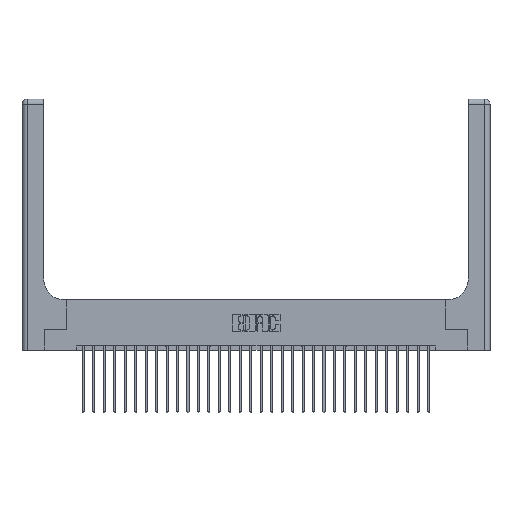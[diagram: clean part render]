
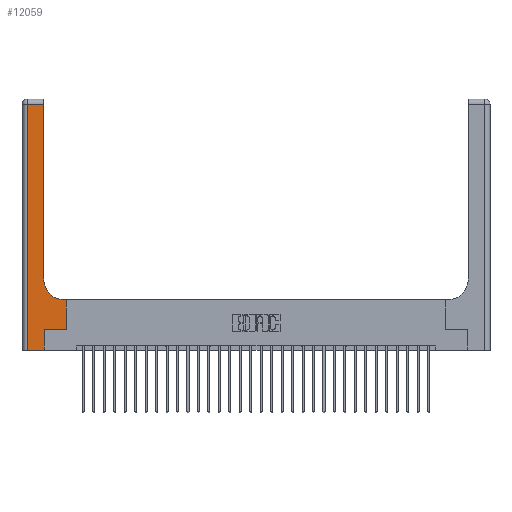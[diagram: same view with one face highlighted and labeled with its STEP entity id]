
A CAD part, top view. The second image highlights one B-rep face of the part: STEP entity #12059.
In plain terms, the highlighted planar face has unit normal (0, 0, 1).
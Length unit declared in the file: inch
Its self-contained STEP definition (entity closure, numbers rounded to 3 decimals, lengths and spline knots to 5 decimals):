
#55 = VECTOR ( 'NONE', #26331, 39.37008 ) ;
#72 = VECTOR ( 'NONE', #21310, 39.37008 ) ;
#436 = ORIENTED_EDGE ( 'NONE', *, *, #23866, .T. ) ;
#714 = DIRECTION ( 'NONE',  ( -1., 0., 0. ) ) ;
#1116 = VECTOR ( 'NONE', #714, 39.37008 ) ;
#1764 = CARTESIAN_POINT ( 'NONE',  ( 0.06, 3., 0.37 ) ) ;
#2154 = LINE ( 'NONE', #19172, #72 ) ;
#3018 = EDGE_CURVE ( 'NONE', #22150, #5124, #15526, .T. ) ;
#3043 = ORIENTED_EDGE ( 'NONE', *, *, #27311, .T. ) ;
#3549 = CARTESIAN_POINT ( 'NONE',  ( 0.26, 0.85, 0.37 ) ) ;
#3781 = CARTESIAN_POINT ( 'NONE',  ( 0.51, 0.85, 0.37 ) ) ;
#4613 = CARTESIAN_POINT ( 'NONE',  ( 0.265, 0., 0.37 ) ) ;
#4993 = DIRECTION ( 'NONE',  ( 0., 1., 0. ) ) ;
#5124 = VERTEX_POINT ( 'NONE', #4613 ) ;
#5157 = CARTESIAN_POINT ( 'NONE',  ( 0.06, 0., 0.37 ) ) ;
#5396 = LINE ( 'NONE', #1764, #17727 ) ;
#5740 = DIRECTION ( 'NONE',  ( 0., 1., 0. ) ) ;
#6293 = ORIENTED_EDGE ( 'NONE', *, *, #20589, .T. ) ;
#6613 = LINE ( 'NONE', #21767, #55 ) ;
#7165 = CARTESIAN_POINT ( 'NONE',  ( 0.26, 0.6, 0.37 ) ) ;
#7364 = CARTESIAN_POINT ( 'NONE',  ( 0.26, 2.94, 0.37 ) ) ;
#7714 = DIRECTION ( 'NONE',  ( 1., 0., 0. ) ) ;
#8319 = ORIENTED_EDGE ( 'NONE', *, *, #24906, .T. ) ;
#8656 = CARTESIAN_POINT ( 'NONE',  ( 0., 3., 0.37 ) ) ;
#9081 = DIRECTION ( 'NONE',  ( -1., 0., 0. ) ) ;
#9503 = ORIENTED_EDGE ( 'NONE', *, *, #3018, .T. ) ;
#11969 = CARTESIAN_POINT ( 'NONE',  ( 0.265, 0.25, 0.37 ) ) ;
#12059 = ADVANCED_FACE ( 'NONE', ( #12365 ), #17555, .F. ) ;
#12365 = FACE_OUTER_BOUND ( 'NONE', #21639, .T. ) ;
#12831 = VERTEX_POINT ( 'NONE', #17011 ) ;
#13484 = LINE ( 'NONE', #26593, #18598 ) ;
#14391 = VERTEX_POINT ( 'NONE', #7364 ) ;
#14544 = VERTEX_POINT ( 'NONE', #11969 ) ;
#14594 = CARTESIAN_POINT ( 'NONE',  ( 0., 0., 0.37 ) ) ;
#14721 = DIRECTION ( 'NONE',  ( 0., 0., -1. ) ) ;
#15526 = LINE ( 'NONE', #14594, #24172 ) ;
#15641 = LINE ( 'NONE', #23110, #21147 ) ;
#15706 = ORIENTED_EDGE ( 'NONE', *, *, #27822, .T. ) ;
#15832 = LINE ( 'NONE', #7165, #1116 ) ;
#15925 = EDGE_CURVE ( 'NONE', #14544, #12831, #6613, .T. ) ;
#17011 = CARTESIAN_POINT ( 'NONE',  ( 0.528, 0.25, 0.37 ) ) ;
#17208 = DIRECTION ( 'NONE',  ( 0., -1., 0. ) ) ;
#17555 = PLANE ( 'NONE',  #25112 ) ;
#17593 = CARTESIAN_POINT ( 'NONE',  ( 0.528, 0.6, 0.37 ) ) ;
#17727 = VECTOR ( 'NONE', #17208, 39.37008 ) ;
#17891 = CIRCLE ( 'NONE', #23063, 0.25 ) ;
#18023 = DIRECTION ( 'NONE',  ( 0., 0., -1. ) ) ;
#18598 = VECTOR ( 'NONE', #9081, 39.37008 ) ;
#19172 = CARTESIAN_POINT ( 'NONE',  ( 0.265, 0., 0.37 ) ) ;
#20398 = ORIENTED_EDGE ( 'NONE', *, *, #15925, .T. ) ;
#20431 = DIRECTION ( 'NONE',  ( -1., 0., 0. ) ) ;
#20589 = EDGE_CURVE ( 'NONE', #26113, #14391, #15641, .T. ) ;
#21147 = VECTOR ( 'NONE', #5740, 39.37008 ) ;
#21310 = DIRECTION ( 'NONE',  ( 0., 1., 0. ) ) ;
#21639 = EDGE_LOOP ( 'NONE', ( #6293, #436, #8319, #9503, #3043, #20398, #26735, #26748, #15706 ) ) ;
#21767 = CARTESIAN_POINT ( 'NONE',  ( 0.265, 0.25, 0.37 ) ) ;
#22150 = VERTEX_POINT ( 'NONE', #5157 ) ;
#22161 = CARTESIAN_POINT ( 'NONE',  ( 0.528, 0.25, 0.37 ) ) ;
#23063 = AXIS2_PLACEMENT_3D ( 'NONE', #3781, #14721, #26095 ) ;
#23110 = CARTESIAN_POINT ( 'NONE',  ( 0.26, 3., 0.37 ) ) ;
#23128 = CARTESIAN_POINT ( 'NONE',  ( 0.51, 0.6, 0.37 ) ) ;
#23279 = EDGE_CURVE ( 'NONE', #12831, #25105, #27937, .T. ) ;
#23689 = VERTEX_POINT ( 'NONE', #23128 ) ;
#23866 = EDGE_CURVE ( 'NONE', #14391, #24365, #13484, .T. ) ;
#23924 = EDGE_CURVE ( 'NONE', #25105, #23689, #15832, .T. ) ;
#24172 = VECTOR ( 'NONE', #7714, 39.37008 ) ;
#24365 = VERTEX_POINT ( 'NONE', #26622 ) ;
#24906 = EDGE_CURVE ( 'NONE', #24365, #22150, #5396, .T. ) ;
#25105 = VERTEX_POINT ( 'NONE', #17593 ) ;
#25112 = AXIS2_PLACEMENT_3D ( 'NONE', #8656, #18023, #20431 ) ;
#26095 = DIRECTION ( 'NONE',  ( 1., 0., 0. ) ) ;
#26113 = VERTEX_POINT ( 'NONE', #3549 ) ;
#26331 = DIRECTION ( 'NONE',  ( 1., 0., 0. ) ) ;
#26570 = VECTOR ( 'NONE', #4993, 39.37008 ) ;
#26593 = CARTESIAN_POINT ( 'NONE',  ( 0., 2.94, 0.37 ) ) ;
#26622 = CARTESIAN_POINT ( 'NONE',  ( 0.06, 2.94, 0.37 ) ) ;
#26735 = ORIENTED_EDGE ( 'NONE', *, *, #23279, .T. ) ;
#26748 = ORIENTED_EDGE ( 'NONE', *, *, #23924, .T. ) ;
#27311 = EDGE_CURVE ( 'NONE', #5124, #14544, #2154, .T. ) ;
#27822 = EDGE_CURVE ( 'NONE', #23689, #26113, #17891, .T. ) ;
#27937 = LINE ( 'NONE', #22161, #26570 ) ;
